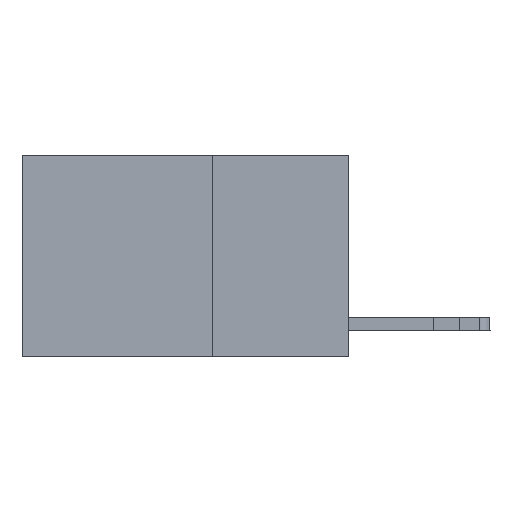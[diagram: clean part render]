
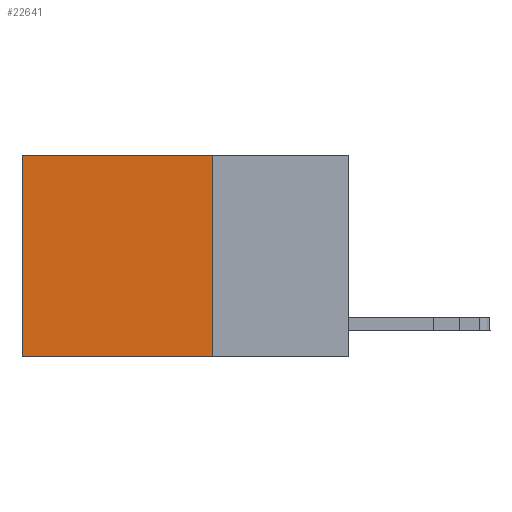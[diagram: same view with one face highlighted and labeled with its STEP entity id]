
A CAD part, left-side view. The second image highlights one B-rep face of the part: STEP entity #22641.
In plain terms, the highlighted planar face has unit normal (-1, 0, 0).
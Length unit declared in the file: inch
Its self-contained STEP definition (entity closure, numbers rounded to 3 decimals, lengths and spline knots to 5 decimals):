
#1032 = CARTESIAN_POINT ( 'NONE',  ( 0.2625, 0.6, -0.37 ) ) ;
#1115 = EDGE_CURVE ( 'NONE', #11253, #20289, #2402, .T. ) ;
#1304 = CARTESIAN_POINT ( 'NONE',  ( 0.2625, 0.25, 0. ) ) ;
#1842 = CARTESIAN_POINT ( 'NONE',  ( 0.2625, 0.25, -0.37 ) ) ;
#2402 = LINE ( 'NONE', #13696, #16359 ) ;
#2792 = CARTESIAN_POINT ( 'NONE',  ( 0.2625, 0.6, 0. ) ) ;
#2976 = EDGE_LOOP ( 'NONE', ( #21934, #19832, #7961, #20648 ) ) ;
#3239 = DIRECTION ( 'NONE',  ( 1., 0., 0. ) ) ;
#4442 = EDGE_CURVE ( 'NONE', #11253, #5099, #10475, .T. ) ;
#5099 = VERTEX_POINT ( 'NONE', #13501 ) ;
#5128 = AXIS2_PLACEMENT_3D ( 'NONE', #6960, #3239, #21705 ) ;
#6960 = CARTESIAN_POINT ( 'NONE',  ( 0.2625, 0.25, 0. ) ) ;
#7258 = DIRECTION ( 'NONE',  ( 0., 0., -1. ) ) ;
#7777 = EDGE_CURVE ( 'NONE', #5099, #14802, #18595, .T. ) ;
#7961 = ORIENTED_EDGE ( 'NONE', *, *, #4442, .F. ) ;
#8369 = DIRECTION ( 'NONE',  ( 0., 1., 0. ) ) ;
#9653 = DIRECTION ( 'NONE',  ( 0., 0., -1. ) ) ;
#10475 = LINE ( 'NONE', #20139, #22819 ) ;
#11253 = VERTEX_POINT ( 'NONE', #1304 ) ;
#11393 = CARTESIAN_POINT ( 'NONE',  ( 0.2625, 0.6, 0. ) ) ;
#12982 = VECTOR ( 'NONE', #18337, 39.37008 ) ;
#13501 = CARTESIAN_POINT ( 'NONE',  ( 0.2625, 0.25, -0.37 ) ) ;
#13696 = CARTESIAN_POINT ( 'NONE',  ( 0.2625, 0.25, 0. ) ) ;
#14284 = PLANE ( 'NONE',  #5128 ) ;
#14802 = VERTEX_POINT ( 'NONE', #1032 ) ;
#16359 = VECTOR ( 'NONE', #8369, 39.37008 ) ;
#16525 = EDGE_CURVE ( 'NONE', #20289, #14802, #16963, .T. ) ;
#16963 = LINE ( 'NONE', #11393, #23539 ) ;
#18337 = DIRECTION ( 'NONE',  ( 0., 1., 0. ) ) ;
#18595 = LINE ( 'NONE', #1842, #12982 ) ;
#19832 = ORIENTED_EDGE ( 'NONE', *, *, #7777, .F. ) ;
#20139 = CARTESIAN_POINT ( 'NONE',  ( 0.2625, 0.25, 0. ) ) ;
#20289 = VERTEX_POINT ( 'NONE', #2792 ) ;
#20648 = ORIENTED_EDGE ( 'NONE', *, *, #1115, .T. ) ;
#21705 = DIRECTION ( 'NONE',  ( 0., 0., -1. ) ) ;
#21934 = ORIENTED_EDGE ( 'NONE', *, *, #16525, .T. ) ;
#22641 = ADVANCED_FACE ( 'NONE', ( #23699 ), #14284, .F. ) ;
#22819 = VECTOR ( 'NONE', #7258, 39.37008 ) ;
#23539 = VECTOR ( 'NONE', #9653, 39.37008 ) ;
#23699 = FACE_OUTER_BOUND ( 'NONE', #2976, .T. ) ;
